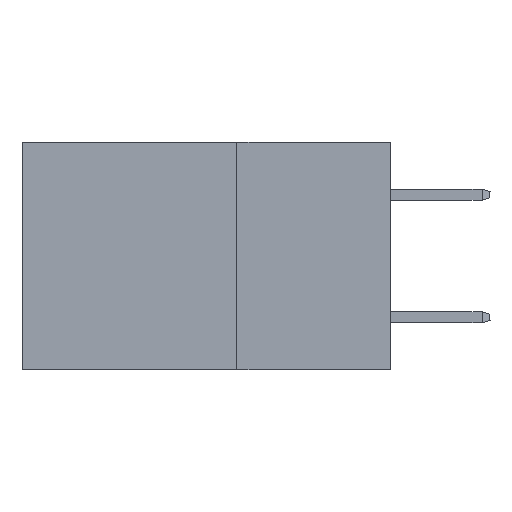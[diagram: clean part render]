
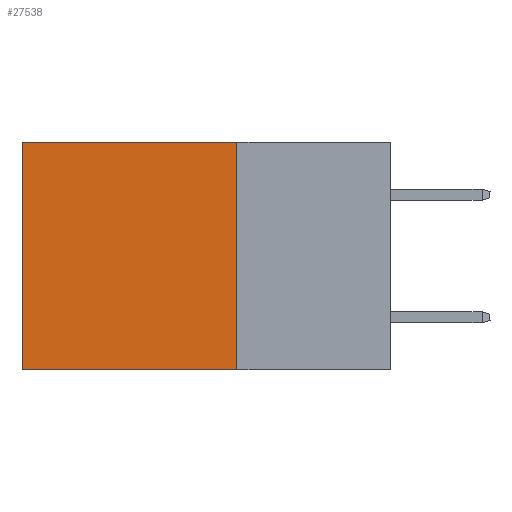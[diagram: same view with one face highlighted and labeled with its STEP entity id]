
A CAD part, left-side view. The second image highlights one B-rep face of the part: STEP entity #27538.
In plain terms, the highlighted planar face has unit normal (-1, 0, 0).
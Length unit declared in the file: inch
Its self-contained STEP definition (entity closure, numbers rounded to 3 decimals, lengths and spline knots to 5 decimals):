
#5102 = DIRECTION ( 'NONE',  ( 1., 0., 0. ) ) ;
#5258 = CARTESIAN_POINT ( 'NONE',  ( 0.2875, 0.25, 0. ) ) ;
#5624 = VERTEX_POINT ( 'NONE', #5258 ) ;
#7073 = ORIENTED_EDGE ( 'NONE', *, *, #24953, .F. ) ;
#8137 = VECTOR ( 'NONE', #34277, 39.37008 ) ;
#8339 = VERTEX_POINT ( 'NONE', #29696 ) ;
#8526 = ORIENTED_EDGE ( 'NONE', *, *, #15538, .T. ) ;
#10778 = VERTEX_POINT ( 'NONE', #37913 ) ;
#10889 = PLANE ( 'NONE',  #28828 ) ;
#11449 = DIRECTION ( 'NONE',  ( 0., 1., 0. ) ) ;
#11482 = FACE_OUTER_BOUND ( 'NONE', #12595, .T. ) ;
#12595 = EDGE_LOOP ( 'NONE', ( #8526, #7073, #22389, #26866 ) ) ;
#13676 = VERTEX_POINT ( 'NONE', #19492 ) ;
#13758 = VECTOR ( 'NONE', #21176, 39.37008 ) ;
#15001 = DIRECTION ( 'NONE',  ( 0., 0., -1. ) ) ;
#15538 = EDGE_CURVE ( 'NONE', #10778, #8339, #23864, .T. ) ;
#16704 = VECTOR ( 'NONE', #11449, 39.37008 ) ;
#19492 = CARTESIAN_POINT ( 'NONE',  ( 0.2875, 0.25, -0.37 ) ) ;
#21176 = DIRECTION ( 'NONE',  ( 0., 1., 0. ) ) ;
#21602 = LINE ( 'NONE', #35820, #13758 ) ;
#22389 = ORIENTED_EDGE ( 'NONE', *, *, #29853, .F. ) ;
#22813 = CARTESIAN_POINT ( 'NONE',  ( 0.2875, 0.25, 0. ) ) ;
#23864 = LINE ( 'NONE', #31346, #8137 ) ;
#24953 = EDGE_CURVE ( 'NONE', #13676, #8339, #32381, .T. ) ;
#25061 = VECTOR ( 'NONE', #15001, 39.37008 ) ;
#25782 = DIRECTION ( 'NONE',  ( 0., 0., -1. ) ) ;
#26866 = ORIENTED_EDGE ( 'NONE', *, *, #33115, .T. ) ;
#27538 = ADVANCED_FACE ( 'NONE', ( #11482 ), #10889, .F. ) ;
#28828 = AXIS2_PLACEMENT_3D ( 'NONE', #22813, #5102, #25782 ) ;
#29696 = CARTESIAN_POINT ( 'NONE',  ( 0.2875, 0.6, -0.37 ) ) ;
#29853 = EDGE_CURVE ( 'NONE', #5624, #13676, #32872, .T. ) ;
#31346 = CARTESIAN_POINT ( 'NONE',  ( 0.2875, 0.6, 0. ) ) ;
#32084 = CARTESIAN_POINT ( 'NONE',  ( 0.2875, 0.25, -0.37 ) ) ;
#32381 = LINE ( 'NONE', #32084, #16704 ) ;
#32872 = LINE ( 'NONE', #35561, #25061 ) ;
#33115 = EDGE_CURVE ( 'NONE', #5624, #10778, #21602, .T. ) ;
#34277 = DIRECTION ( 'NONE',  ( 0., 0., -1. ) ) ;
#35561 = CARTESIAN_POINT ( 'NONE',  ( 0.2875, 0.25, 0. ) ) ;
#35820 = CARTESIAN_POINT ( 'NONE',  ( 0.2875, 0.25, 0. ) ) ;
#37913 = CARTESIAN_POINT ( 'NONE',  ( 0.2875, 0.6, 0. ) ) ;
